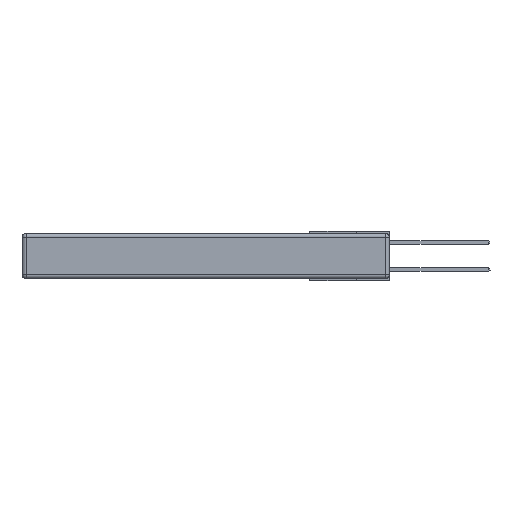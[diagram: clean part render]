
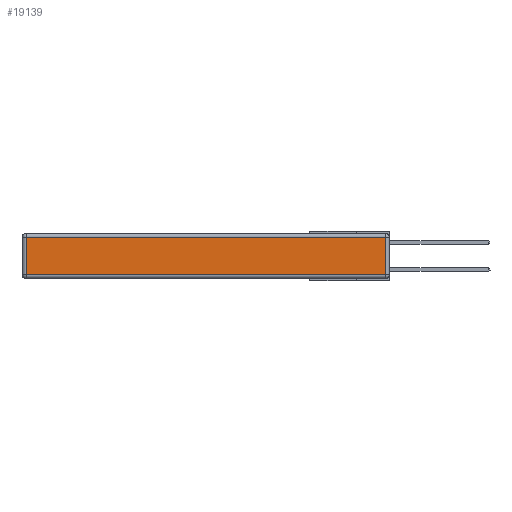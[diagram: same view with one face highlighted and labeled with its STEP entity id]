
A CAD part, left-side view. The second image highlights one B-rep face of the part: STEP entity #19139.
In plain terms, the highlighted planar face has unit normal (-1, 0, 0).
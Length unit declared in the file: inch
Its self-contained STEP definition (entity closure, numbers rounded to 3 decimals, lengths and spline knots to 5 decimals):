
#3826 = EDGE_CURVE ( 'NONE', #25414, #24370, #13189, .T. ) ;
#4653 = CARTESIAN_POINT ( 'NONE',  ( 0., 2.72, -0.343 ) ) ;
#6707 = VECTOR ( 'NONE', #22530, 39.37008 ) ;
#10501 = CARTESIAN_POINT ( 'NONE',  ( 0., 2.72, -0.313 ) ) ;
#10535 = ORIENTED_EDGE ( 'NONE', *, *, #10948, .T. ) ;
#10948 = EDGE_CURVE ( 'NONE', #24370, #18447, #11418, .T. ) ;
#11409 = CARTESIAN_POINT ( 'NONE',  ( 0., 0., -0.313 ) ) ;
#11418 = LINE ( 'NONE', #11409, #21839 ) ;
#11676 = PLANE ( 'NONE',  #27305 ) ;
#12799 = VECTOR ( 'NONE', #30480, 39.37008 ) ;
#13189 = LINE ( 'NONE', #4653, #14281 ) ;
#13601 = DIRECTION ( 'NONE',  ( 0., -1., 0. ) ) ;
#14281 = VECTOR ( 'NONE', #23708, 39.37008 ) ;
#17335 = EDGE_LOOP ( 'NONE', ( #10535, #22945, #20311, #30529 ) ) ;
#17493 = EDGE_CURVE ( 'NONE', #18447, #22917, #20135, .T. ) ;
#17634 = LINE ( 'NONE', #25869, #12799 ) ;
#17751 = CARTESIAN_POINT ( 'NONE',  ( 0., 0.03, -0.343 ) ) ;
#18447 = VERTEX_POINT ( 'NONE', #18802 ) ;
#18580 = CARTESIAN_POINT ( 'NONE',  ( 0., 2.72, -0.03 ) ) ;
#18802 = CARTESIAN_POINT ( 'NONE',  ( 0., 0.03, -0.313 ) ) ;
#18977 = DIRECTION ( 'NONE',  ( -1., 0., 0. ) ) ;
#19139 = ADVANCED_FACE ( 'NONE', ( #28966 ), #11676, .T. ) ;
#20135 = LINE ( 'NONE', #17751, #6707 ) ;
#20311 = ORIENTED_EDGE ( 'NONE', *, *, #28673, .T. ) ;
#21839 = VECTOR ( 'NONE', #13601, 39.37008 ) ;
#22530 = DIRECTION ( 'NONE',  ( 0., 0., 1. ) ) ;
#22917 = VERTEX_POINT ( 'NONE', #29752 ) ;
#22945 = ORIENTED_EDGE ( 'NONE', *, *, #17493, .T. ) ;
#23708 = DIRECTION ( 'NONE',  ( 0., 0., -1. ) ) ;
#24370 = VERTEX_POINT ( 'NONE', #10501 ) ;
#25414 = VERTEX_POINT ( 'NONE', #18580 ) ;
#25869 = CARTESIAN_POINT ( 'NONE',  ( 0., 2.75, -0.03 ) ) ;
#25922 = CARTESIAN_POINT ( 'NONE',  ( 0., 0., -0.343 ) ) ;
#27305 = AXIS2_PLACEMENT_3D ( 'NONE', #25922, #18977, #30839 ) ;
#28673 = EDGE_CURVE ( 'NONE', #22917, #25414, #17634, .T. ) ;
#28966 = FACE_OUTER_BOUND ( 'NONE', #17335, .T. ) ;
#29752 = CARTESIAN_POINT ( 'NONE',  ( 0., 0.03, -0.03 ) ) ;
#30480 = DIRECTION ( 'NONE',  ( 0., 1., 0. ) ) ;
#30529 = ORIENTED_EDGE ( 'NONE', *, *, #3826, .T. ) ;
#30839 = DIRECTION ( 'NONE',  ( 0., 0., 1. ) ) ;
